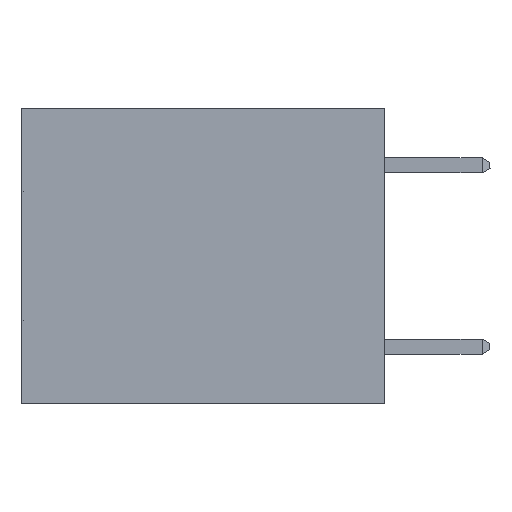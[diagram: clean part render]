
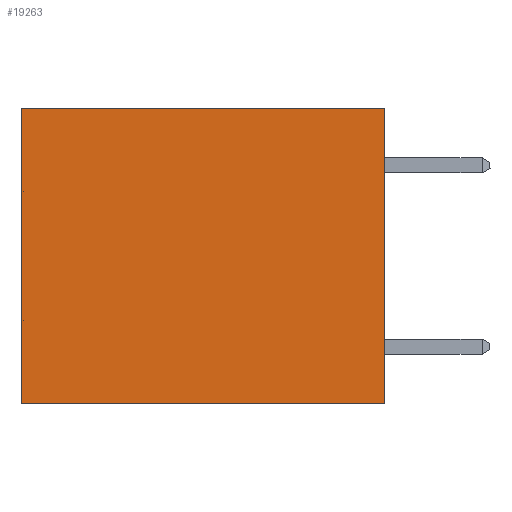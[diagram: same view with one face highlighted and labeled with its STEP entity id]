
A CAD part, left-side view. The second image highlights one B-rep face of the part: STEP entity #19263.
In plain terms, the highlighted planar face has unit normal (-1, 0, 0).
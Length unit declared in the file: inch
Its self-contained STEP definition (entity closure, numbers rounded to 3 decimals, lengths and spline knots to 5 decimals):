
#372 = CARTESIAN_POINT ( 'NONE',  ( 0.3165, 0.6, -0.49 ) ) ;
#692 = CARTESIAN_POINT ( 'NONE',  ( 0.3165, 0., 0. ) ) ;
#1473 = CARTESIAN_POINT ( 'NONE',  ( 0.3165, 0., 0. ) ) ;
#2012 = CARTESIAN_POINT ( 'NONE',  ( 0.3165, 0., -0.49 ) ) ;
#3245 = AXIS2_PLACEMENT_3D ( 'NONE', #17397, #30111, #25033 ) ;
#3424 = VECTOR ( 'NONE', #13157, 39.37008 ) ;
#4843 = CARTESIAN_POINT ( 'NONE',  ( 0.3165, 0., -0.49 ) ) ;
#5207 = CARTESIAN_POINT ( 'NONE',  ( 0.3165, 0.6, -0.49 ) ) ;
#5550 = DIRECTION ( 'NONE',  ( 0., 1., 0. ) ) ;
#5716 = EDGE_CURVE ( 'NONE', #19829, #23381, #9111, .T. ) ;
#6183 = VERTEX_POINT ( 'NONE', #1473 ) ;
#7073 = ORIENTED_EDGE ( 'NONE', *, *, #22560, .T. ) ;
#9111 = LINE ( 'NONE', #5207, #3424 ) ;
#9310 = VECTOR ( 'NONE', #26362, 39.37008 ) ;
#9926 = LINE ( 'NONE', #4843, #29711 ) ;
#13157 = DIRECTION ( 'NONE',  ( 0., 0., -1. ) ) ;
#13487 = VECTOR ( 'NONE', #5550, 39.37008 ) ;
#14399 = FACE_OUTER_BOUND ( 'NONE', #30248, .T. ) ;
#14401 = EDGE_CURVE ( 'NONE', #6183, #14953, #9926, .T. ) ;
#14953 = VERTEX_POINT ( 'NONE', #2012 ) ;
#15531 = DIRECTION ( 'NONE',  ( 0., 0., -1. ) ) ;
#15887 = CARTESIAN_POINT ( 'NONE',  ( 0.3165, 0., -0.49 ) ) ;
#17397 = CARTESIAN_POINT ( 'NONE',  ( 0.3165, 0., -0.49 ) ) ;
#19263 = ADVANCED_FACE ( 'NONE', ( #14399 ), #22654, .F. ) ;
#19829 = VERTEX_POINT ( 'NONE', #25059 ) ;
#20344 = LINE ( 'NONE', #15887, #13487 ) ;
#21519 = EDGE_CURVE ( 'NONE', #14953, #23381, #20344, .T. ) ;
#22560 = EDGE_CURVE ( 'NONE', #6183, #19829, #29551, .T. ) ;
#22583 = ORIENTED_EDGE ( 'NONE', *, *, #21519, .F. ) ;
#22654 = PLANE ( 'NONE',  #3245 ) ;
#23381 = VERTEX_POINT ( 'NONE', #372 ) ;
#25033 = DIRECTION ( 'NONE',  ( 0., 0., -1. ) ) ;
#25059 = CARTESIAN_POINT ( 'NONE',  ( 0.3165, 0.6, 0. ) ) ;
#26362 = DIRECTION ( 'NONE',  ( 0., 1., 0. ) ) ;
#27837 = ORIENTED_EDGE ( 'NONE', *, *, #5716, .T. ) ;
#29551 = LINE ( 'NONE', #692, #9310 ) ;
#29711 = VECTOR ( 'NONE', #15531, 39.37008 ) ;
#30111 = DIRECTION ( 'NONE',  ( 1., 0., 0. ) ) ;
#30248 = EDGE_LOOP ( 'NONE', ( #27837, #22583, #30652, #7073 ) ) ;
#30652 = ORIENTED_EDGE ( 'NONE', *, *, #14401, .F. ) ;
